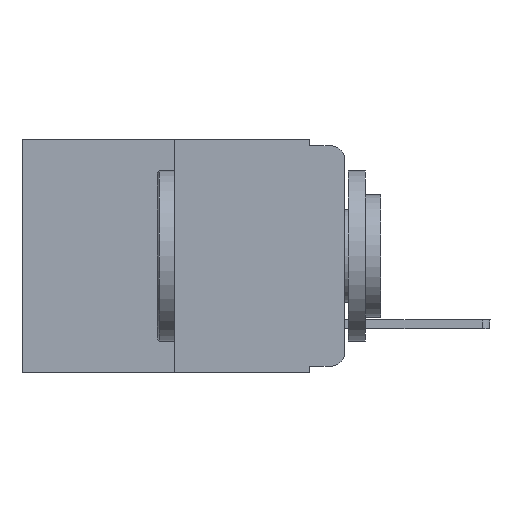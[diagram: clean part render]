
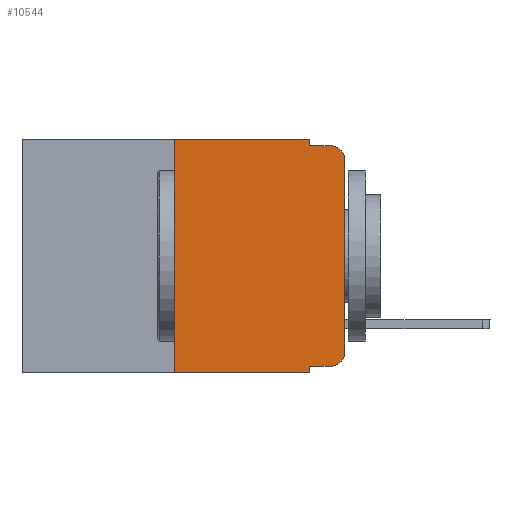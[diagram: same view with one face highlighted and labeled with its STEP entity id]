
A CAD part, left-side view. The second image highlights one B-rep face of the part: STEP entity #10544.
In plain terms, the highlighted planar face has unit normal (-1, 0, 0).
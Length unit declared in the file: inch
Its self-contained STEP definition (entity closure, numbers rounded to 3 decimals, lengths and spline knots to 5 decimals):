
#562 = CARTESIAN_POINT ( 'NONE',  ( 0., 0., -0.03 ) ) ;
#764 = ORIENTED_EDGE ( 'NONE', *, *, #3971, .F. ) ;
#1029 = ORIENTED_EDGE ( 'NONE', *, *, #10305, .T. ) ;
#1194 = VECTOR ( 'NONE', #5387, 39.37008 ) ;
#1395 = ORIENTED_EDGE ( 'NONE', *, *, #4057, .F. ) ;
#1496 = VERTEX_POINT ( 'NONE', #562 ) ;
#1649 = CARTESIAN_POINT ( 'NONE',  ( 0., 0.473, 0. ) ) ;
#1743 = VERTEX_POINT ( 'NONE', #2453 ) ;
#1877 = LINE ( 'NONE', #19837, #1194 ) ;
#2403 = CARTESIAN_POINT ( 'NONE',  ( 0., 0.473, 0. ) ) ;
#2453 = CARTESIAN_POINT ( 'NONE',  ( 0., 0.02, -0.01 ) ) ;
#2687 = ORIENTED_EDGE ( 'NONE', *, *, #14796, .F. ) ;
#2731 = DIRECTION ( 'NONE',  ( 0., 0., -1. ) ) ;
#3091 = CARTESIAN_POINT ( 'NONE',  ( 0., 0.25, -0.343 ) ) ;
#3272 = CARTESIAN_POINT ( 'NONE',  ( 0., 0.25, 0. ) ) ;
#3504 = VERTEX_POINT ( 'NONE', #3272 ) ;
#3665 = EDGE_CURVE ( 'NONE', #15534, #9362, #8854, .T. ) ;
#3678 = DIRECTION ( 'NONE',  ( -1., 0., 0. ) ) ;
#3971 = EDGE_CURVE ( 'NONE', #17436, #1743, #1877, .T. ) ;
#4057 = EDGE_CURVE ( 'NONE', #15448, #3504, #9148, .T. ) ;
#4187 = DIRECTION ( 'NONE',  ( 0., 0., -1. ) ) ;
#4403 = LINE ( 'NONE', #7451, #14580 ) ;
#5010 = VECTOR ( 'NONE', #9120, 39.37008 ) ;
#5387 = DIRECTION ( 'NONE',  ( 0., -1., 0. ) ) ;
#5560 = LINE ( 'NONE', #8716, #8481 ) ;
#6832 = VECTOR ( 'NONE', #2731, 39.37008 ) ;
#6859 = DIRECTION ( 'NONE',  ( -1., 0., 0. ) ) ;
#7231 = AXIS2_PLACEMENT_3D ( 'NONE', #13385, #3678, #18142 ) ;
#7250 = DIRECTION ( 'NONE',  ( 0., 0., 1. ) ) ;
#7451 = CARTESIAN_POINT ( 'NONE',  ( 0., 0.051, 0. ) ) ;
#7946 = VERTEX_POINT ( 'NONE', #15880 ) ;
#8161 = CARTESIAN_POINT ( 'NONE',  ( 0., 0.473, -0.343 ) ) ;
#8385 = AXIS2_PLACEMENT_3D ( 'NONE', #8446, #6859, #19851 ) ;
#8446 = CARTESIAN_POINT ( 'NONE',  ( 0., 0.02, -0.03 ) ) ;
#8481 = VECTOR ( 'NONE', #12082, 39.37008 ) ;
#8716 = CARTESIAN_POINT ( 'NONE',  ( 0., 0., 0. ) ) ;
#8854 = LINE ( 'NONE', #15511, #6832 ) ;
#9120 = DIRECTION ( 'NONE',  ( 0., -1., 0. ) ) ;
#9148 = LINE ( 'NONE', #10431, #17398 ) ;
#9362 = VERTEX_POINT ( 'NONE', #14828 ) ;
#9469 = CARTESIAN_POINT ( 'NONE',  ( 0., 0.051, -0.01 ) ) ;
#10099 = DIRECTION ( 'NONE',  ( 0., 0., -1. ) ) ;
#10305 = EDGE_CURVE ( 'NONE', #1496, #1743, #17490, .T. ) ;
#10431 = CARTESIAN_POINT ( 'NONE',  ( 0., 0.25, 0. ) ) ;
#10443 = FACE_OUTER_BOUND ( 'NONE', #10601, .T. ) ;
#10544 = ADVANCED_FACE ( 'NONE', ( #10443 ), #16871, .F. ) ;
#10601 = EDGE_LOOP ( 'NONE', ( #13733, #1029, #764, #2687, #13091, #1395, #18467, #15146, #10716, #17459 ) ) ;
#10716 = ORIENTED_EDGE ( 'NONE', *, *, #10931, .T. ) ;
#10870 = VECTOR ( 'NONE', #13018, 39.37008 ) ;
#10931 = EDGE_CURVE ( 'NONE', #15534, #12503, #15656, .T. ) ;
#11341 = LINE ( 'NONE', #8161, #10870 ) ;
#12082 = DIRECTION ( 'NONE',  ( 0., 0., 1. ) ) ;
#12503 = VERTEX_POINT ( 'NONE', #19808 ) ;
#12537 = EDGE_CURVE ( 'NONE', #3504, #7946, #13148, .T. ) ;
#13018 = DIRECTION ( 'NONE',  ( 0., -1., 0. ) ) ;
#13091 = ORIENTED_EDGE ( 'NONE', *, *, #12537, .F. ) ;
#13148 = LINE ( 'NONE', #1649, #17188 ) ;
#13385 = CARTESIAN_POINT ( 'NONE',  ( 0., 0.02, -0.313 ) ) ;
#13733 = ORIENTED_EDGE ( 'NONE', *, *, #13941, .T. ) ;
#13941 = EDGE_CURVE ( 'NONE', #16423, #1496, #5560, .T. ) ;
#14304 = EDGE_CURVE ( 'NONE', #15448, #9362, #11341, .T. ) ;
#14580 = VECTOR ( 'NONE', #4187, 39.37008 ) ;
#14796 = EDGE_CURVE ( 'NONE', #7946, #17436, #4403, .T. ) ;
#14828 = CARTESIAN_POINT ( 'NONE',  ( 0., 0.051, -0.343 ) ) ;
#14920 = CARTESIAN_POINT ( 'NONE',  ( 0., 0.051, -0.333 ) ) ;
#15146 = ORIENTED_EDGE ( 'NONE', *, *, #3665, .F. ) ;
#15448 = VERTEX_POINT ( 'NONE', #3091 ) ;
#15511 = CARTESIAN_POINT ( 'NONE',  ( 0., 0.051, 0. ) ) ;
#15534 = VERTEX_POINT ( 'NONE', #14920 ) ;
#15556 = CARTESIAN_POINT ( 'NONE',  ( 0., 0.051, -0.333 ) ) ;
#15656 = LINE ( 'NONE', #15556, #5010 ) ;
#15880 = CARTESIAN_POINT ( 'NONE',  ( 0., 0.051, 0. ) ) ;
#16338 = CIRCLE ( 'NONE', #7231, 0.02 ) ;
#16423 = VERTEX_POINT ( 'NONE', #17097 ) ;
#16871 = PLANE ( 'NONE',  #17152 ) ;
#17097 = CARTESIAN_POINT ( 'NONE',  ( 0., 0., -0.313 ) ) ;
#17152 = AXIS2_PLACEMENT_3D ( 'NONE', #2403, #18000, #10099 ) ;
#17188 = VECTOR ( 'NONE', #19591, 39.37008 ) ;
#17398 = VECTOR ( 'NONE', #7250, 39.37008 ) ;
#17436 = VERTEX_POINT ( 'NONE', #9469 ) ;
#17459 = ORIENTED_EDGE ( 'NONE', *, *, #18313, .T. ) ;
#17490 = CIRCLE ( 'NONE', #8385, 0.02 ) ;
#18000 = DIRECTION ( 'NONE',  ( 1., 0., 0. ) ) ;
#18142 = DIRECTION ( 'NONE',  ( 0., 0., -1. ) ) ;
#18313 = EDGE_CURVE ( 'NONE', #12503, #16423, #16338, .T. ) ;
#18467 = ORIENTED_EDGE ( 'NONE', *, *, #14304, .T. ) ;
#19591 = DIRECTION ( 'NONE',  ( 0., -1., 0. ) ) ;
#19808 = CARTESIAN_POINT ( 'NONE',  ( 0., 0.02, -0.333 ) ) ;
#19837 = CARTESIAN_POINT ( 'NONE',  ( 0., 0.051, -0.01 ) ) ;
#19851 = DIRECTION ( 'NONE',  ( 0., 0., -1. ) ) ;
